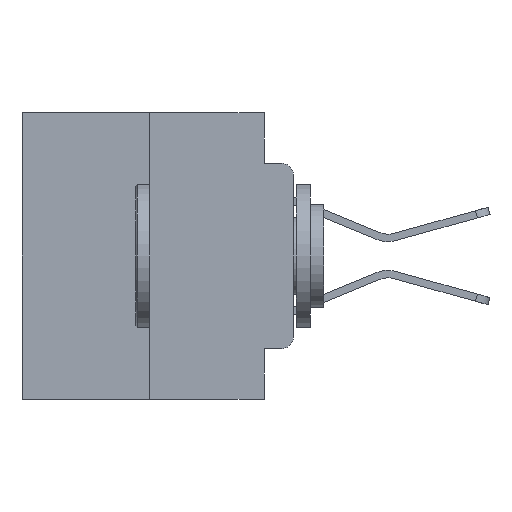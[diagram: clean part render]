
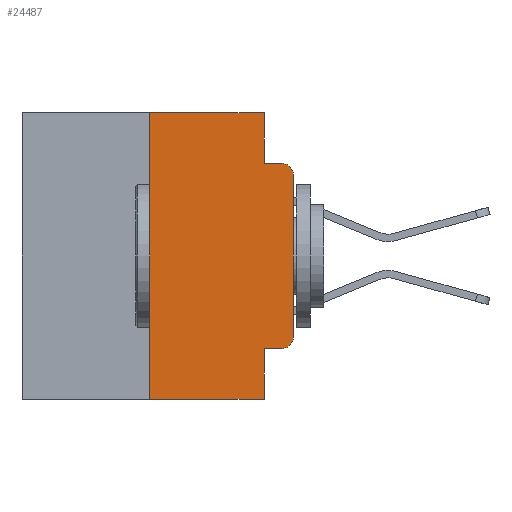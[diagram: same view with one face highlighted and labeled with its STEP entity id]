
A CAD part, left-side view. The second image highlights one B-rep face of the part: STEP entity #24487.
In plain terms, the highlighted planar face has unit normal (-1, 0, 0).
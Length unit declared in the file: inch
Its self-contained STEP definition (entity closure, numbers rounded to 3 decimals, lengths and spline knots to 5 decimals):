
#488 = LINE ( 'NONE', #20894, #11060 ) ;
#557 = AXIS2_PLACEMENT_3D ( 'NONE', #27154, #14519, #1835 ) ;
#1084 = EDGE_CURVE ( 'NONE', #25634, #18959, #7326, .T. ) ;
#1835 = DIRECTION ( 'NONE',  ( 0., 0., -1. ) ) ;
#1913 = EDGE_CURVE ( 'NONE', #17555, #22356, #18573, .T. ) ;
#2444 = DIRECTION ( 'NONE',  ( 0., 0., 1. ) ) ;
#3264 = AXIS2_PLACEMENT_3D ( 'NONE', #6882, #10539, #11068 ) ;
#3348 = EDGE_CURVE ( 'NONE', #10234, #17555, #6534, .T. ) ;
#3457 = ORIENTED_EDGE ( 'NONE', *, *, #1084, .F. ) ;
#3491 = VERTEX_POINT ( 'NONE', #17516 ) ;
#3693 = CARTESIAN_POINT ( 'NONE',  ( 0., 0.051, 0. ) ) ;
#4083 = CARTESIAN_POINT ( 'NONE',  ( 0., 0., -0.1085 ) ) ;
#4109 = VERTEX_POINT ( 'NONE', #13173 ) ;
#4571 = CARTESIAN_POINT ( 'NONE',  ( 0., 0.25, 0. ) ) ;
#5573 = DIRECTION ( 'NONE',  ( 0., -1., 0. ) ) ;
#5759 = ORIENTED_EDGE ( 'NONE', *, *, #6151, .F. ) ;
#6151 = EDGE_CURVE ( 'NONE', #10234, #4109, #8345, .T. ) ;
#6375 = LINE ( 'NONE', #16268, #22658 ) ;
#6520 = VECTOR ( 'NONE', #2444, 39.37008 ) ;
#6534 = LINE ( 'NONE', #15906, #17171 ) ;
#6860 = FACE_OUTER_BOUND ( 'NONE', #13059, .T. ) ;
#6882 = CARTESIAN_POINT ( 'NONE',  ( 0., 0.02, -0.3915 ) ) ;
#7326 = LINE ( 'NONE', #23171, #22949 ) ;
#8174 = PLANE ( 'NONE',  #16994 ) ;
#8345 = LINE ( 'NONE', #22557, #14026 ) ;
#8994 = EDGE_CURVE ( 'NONE', #21753, #25634, #12179, .T. ) ;
#9436 = VECTOR ( 'NONE', #14005, 39.37008 ) ;
#10234 = VERTEX_POINT ( 'NONE', #23675 ) ;
#10327 = DIRECTION ( 'NONE',  ( 1., 0., 0. ) ) ;
#10343 = ORIENTED_EDGE ( 'NONE', *, *, #21800, .T. ) ;
#10411 = VERTEX_POINT ( 'NONE', #22207 ) ;
#10539 = DIRECTION ( 'NONE',  ( -1., 0., 0. ) ) ;
#11060 = VECTOR ( 'NONE', #23058, 39.37008 ) ;
#11068 = DIRECTION ( 'NONE',  ( 0., 0., -1. ) ) ;
#11852 = EDGE_CURVE ( 'NONE', #18959, #10411, #18856, .T. ) ;
#11854 = CARTESIAN_POINT ( 'NONE',  ( 0., 0., 0. ) ) ;
#12179 = LINE ( 'NONE', #4571, #6520 ) ;
#12292 = DIRECTION ( 'NONE',  ( 0., -1., 0. ) ) ;
#12553 = CIRCLE ( 'NONE', #557, 0.02 ) ;
#12559 = VECTOR ( 'NONE', #20621, 39.37008 ) ;
#13059 = EDGE_LOOP ( 'NONE', ( #10343, #23969, #16695, #17035, #3457, #20999, #20682, #5759, #17064, #19692 ) ) ;
#13173 = CARTESIAN_POINT ( 'NONE',  ( 0., 0.051, -0.5 ) ) ;
#13972 = CARTESIAN_POINT ( 'NONE',  ( 0., 0.25, 0. ) ) ;
#14005 = DIRECTION ( 'NONE',  ( 0., 0., 1. ) ) ;
#14026 = VECTOR ( 'NONE', #24658, 39.37008 ) ;
#14519 = DIRECTION ( 'NONE',  ( -1., 0., 0. ) ) ;
#14686 = EDGE_CURVE ( 'NONE', #10411, #3491, #488, .T. ) ;
#15906 = CARTESIAN_POINT ( 'NONE',  ( 0., 0.051, -0.4115 ) ) ;
#15952 = CARTESIAN_POINT ( 'NONE',  ( 0., 0.25, -0.5 ) ) ;
#16268 = CARTESIAN_POINT ( 'NONE',  ( 0., 0.473, -0.5 ) ) ;
#16478 = CARTESIAN_POINT ( 'NONE',  ( 0., 0.02, -0.4115 ) ) ;
#16676 = CARTESIAN_POINT ( 'NONE',  ( 0., 0.051, 0. ) ) ;
#16695 = ORIENTED_EDGE ( 'NONE', *, *, #14686, .F. ) ;
#16994 = AXIS2_PLACEMENT_3D ( 'NONE', #27134, #10327, #25135 ) ;
#17035 = ORIENTED_EDGE ( 'NONE', *, *, #11852, .F. ) ;
#17064 = ORIENTED_EDGE ( 'NONE', *, *, #3348, .T. ) ;
#17171 = VECTOR ( 'NONE', #5573, 39.37008 ) ;
#17516 = CARTESIAN_POINT ( 'NONE',  ( 0., 0.02, -0.0885 ) ) ;
#17555 = VERTEX_POINT ( 'NONE', #16478 ) ;
#18390 = DIRECTION ( 'NONE',  ( 0., -1., 0. ) ) ;
#18573 = CIRCLE ( 'NONE', #3264, 0.02 ) ;
#18856 = LINE ( 'NONE', #3693, #12559 ) ;
#18949 = EDGE_CURVE ( 'NONE', #23856, #3491, #12553, .T. ) ;
#18959 = VERTEX_POINT ( 'NONE', #16676 ) ;
#19692 = ORIENTED_EDGE ( 'NONE', *, *, #1913, .T. ) ;
#20264 = CARTESIAN_POINT ( 'NONE',  ( 0., 0., -0.3915 ) ) ;
#20621 = DIRECTION ( 'NONE',  ( 0., 0., -1. ) ) ;
#20682 = ORIENTED_EDGE ( 'NONE', *, *, #23068, .T. ) ;
#20894 = CARTESIAN_POINT ( 'NONE',  ( 0., 0.051, -0.0885 ) ) ;
#20999 = ORIENTED_EDGE ( 'NONE', *, *, #8994, .F. ) ;
#21753 = VERTEX_POINT ( 'NONE', #15952 ) ;
#21800 = EDGE_CURVE ( 'NONE', #22356, #23856, #26323, .T. ) ;
#22207 = CARTESIAN_POINT ( 'NONE',  ( 0., 0.051, -0.0885 ) ) ;
#22356 = VERTEX_POINT ( 'NONE', #20264 ) ;
#22557 = CARTESIAN_POINT ( 'NONE',  ( 0., 0.051, 0. ) ) ;
#22658 = VECTOR ( 'NONE', #18390, 39.37008 ) ;
#22949 = VECTOR ( 'NONE', #12292, 39.37008 ) ;
#23058 = DIRECTION ( 'NONE',  ( 0., -1., 0. ) ) ;
#23068 = EDGE_CURVE ( 'NONE', #21753, #4109, #6375, .T. ) ;
#23171 = CARTESIAN_POINT ( 'NONE',  ( 0., 0.473, 0. ) ) ;
#23675 = CARTESIAN_POINT ( 'NONE',  ( 0., 0.051, -0.4115 ) ) ;
#23856 = VERTEX_POINT ( 'NONE', #4083 ) ;
#23969 = ORIENTED_EDGE ( 'NONE', *, *, #18949, .T. ) ;
#24487 = ADVANCED_FACE ( 'NONE', ( #6860 ), #8174, .F. ) ;
#24658 = DIRECTION ( 'NONE',  ( 0., 0., -1. ) ) ;
#25135 = DIRECTION ( 'NONE',  ( 0., 0., -1. ) ) ;
#25634 = VERTEX_POINT ( 'NONE', #13972 ) ;
#26323 = LINE ( 'NONE', #11854, #9436 ) ;
#27134 = CARTESIAN_POINT ( 'NONE',  ( 0., 0.473, 0. ) ) ;
#27154 = CARTESIAN_POINT ( 'NONE',  ( 0., 0.02, -0.1085 ) ) ;
